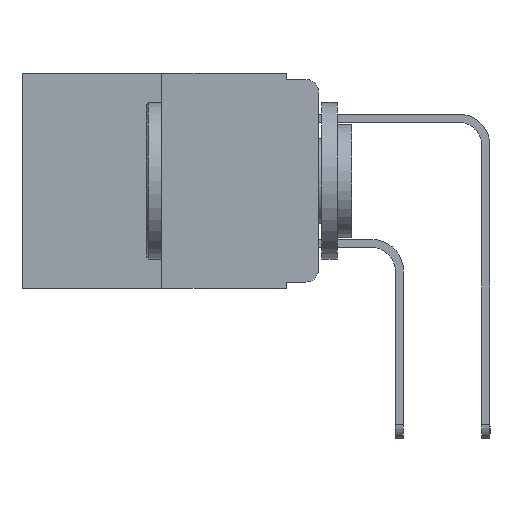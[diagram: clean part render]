
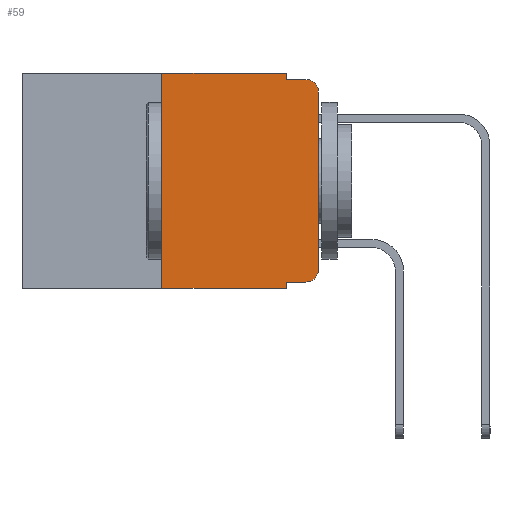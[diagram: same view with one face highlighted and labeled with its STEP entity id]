
A CAD part, left-side view. The second image highlights one B-rep face of the part: STEP entity #59.
In plain terms, the highlighted planar face has unit normal (-1, 0, 0).
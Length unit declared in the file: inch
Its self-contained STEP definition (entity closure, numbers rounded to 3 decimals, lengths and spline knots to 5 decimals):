
#59 = ADVANCED_FACE ( 'NONE', ( #5841 ), #3660, .F. ) ;
#407 = AXIS2_PLACEMENT_3D ( 'NONE', #15184, #13256, #22876 ) ;
#498 = CARTESIAN_POINT ( 'NONE',  ( 0., 0., -0.03 ) ) ;
#936 = CARTESIAN_POINT ( 'NONE',  ( 0., 0.02, -0.333 ) ) ;
#998 = DIRECTION ( 'NONE',  ( 0., 0., -1. ) ) ;
#1811 = EDGE_CURVE ( 'NONE', #6696, #3838, #9662, .T. ) ;
#2507 = CIRCLE ( 'NONE', #14789, 0.02 ) ;
#2534 = VERTEX_POINT ( 'NONE', #14826 ) ;
#2669 = CARTESIAN_POINT ( 'NONE',  ( 0., 0.051, 0. ) ) ;
#2766 = VERTEX_POINT ( 'NONE', #12106 ) ;
#3660 = PLANE ( 'NONE',  #18460 ) ;
#3807 = CARTESIAN_POINT ( 'NONE',  ( 0., 0.02, -0.313 ) ) ;
#3838 = VERTEX_POINT ( 'NONE', #12809 ) ;
#4015 = VECTOR ( 'NONE', #14456, 39.37008 ) ;
#4100 = ORIENTED_EDGE ( 'NONE', *, *, #6868, .T. ) ;
#4613 = VERTEX_POINT ( 'NONE', #936 ) ;
#4682 = CARTESIAN_POINT ( 'NONE',  ( 0., 0., -0.313 ) ) ;
#5069 = LINE ( 'NONE', #18771, #22053 ) ;
#5099 = EDGE_CURVE ( 'NONE', #6022, #4613, #18211, .T. ) ;
#5583 = EDGE_CURVE ( 'NONE', #6022, #3838, #8552, .T. ) ;
#5776 = VERTEX_POINT ( 'NONE', #4682 ) ;
#5841 = FACE_OUTER_BOUND ( 'NONE', #8766, .T. ) ;
#6022 = VERTEX_POINT ( 'NONE', #17378 ) ;
#6070 = LINE ( 'NONE', #13870, #11898 ) ;
#6507 = CARTESIAN_POINT ( 'NONE',  ( 0., 0.051, -0.01 ) ) ;
#6696 = VERTEX_POINT ( 'NONE', #12805 ) ;
#6868 = EDGE_CURVE ( 'NONE', #5776, #18580, #9602, .T. ) ;
#7466 = DIRECTION ( 'NONE',  ( 0., -1., 0. ) ) ;
#7610 = EDGE_CURVE ( 'NONE', #14787, #20910, #5069, .T. ) ;
#7739 = ORIENTED_EDGE ( 'NONE', *, *, #12053, .T. ) ;
#7995 = CARTESIAN_POINT ( 'NONE',  ( 0., 0.473, 0. ) ) ;
#8552 = LINE ( 'NONE', #2669, #16216 ) ;
#8599 = ORIENTED_EDGE ( 'NONE', *, *, #16244, .F. ) ;
#8720 = CARTESIAN_POINT ( 'NONE',  ( 0., 0.051, -0.333 ) ) ;
#8761 = CARTESIAN_POINT ( 'NONE',  ( 0., 0.051, 0. ) ) ;
#8766 = EDGE_LOOP ( 'NONE', ( #4100, #14458, #16681, #8599, #20989, #21946, #22911, #22703, #16181, #7739 ) ) ;
#9048 = CARTESIAN_POINT ( 'NONE',  ( 0., 0.051, 0. ) ) ;
#9602 = LINE ( 'NONE', #21250, #19546 ) ;
#9662 = LINE ( 'NONE', #23233, #20066 ) ;
#11454 = DIRECTION ( 'NONE',  ( 0., 0., -1. ) ) ;
#11843 = CIRCLE ( 'NONE', #407, 0.02 ) ;
#11898 = VECTOR ( 'NONE', #21705, 39.37008 ) ;
#12053 = EDGE_CURVE ( 'NONE', #4613, #5776, #2507, .T. ) ;
#12106 = CARTESIAN_POINT ( 'NONE',  ( 0., 0.051, -0.01 ) ) ;
#12388 = VECTOR ( 'NONE', #22313, 39.37008 ) ;
#12805 = CARTESIAN_POINT ( 'NONE',  ( 0., 0.25, -0.343 ) ) ;
#12809 = CARTESIAN_POINT ( 'NONE',  ( 0., 0.051, -0.343 ) ) ;
#13256 = DIRECTION ( 'NONE',  ( -1., 0., 0. ) ) ;
#13870 = CARTESIAN_POINT ( 'NONE',  ( 0., 0.25, 0. ) ) ;
#14456 = DIRECTION ( 'NONE',  ( 0., -1., 0. ) ) ;
#14458 = ORIENTED_EDGE ( 'NONE', *, *, #20421, .T. ) ;
#14543 = DIRECTION ( 'NONE',  ( 0., -1., 0. ) ) ;
#14787 = VERTEX_POINT ( 'NONE', #20457 ) ;
#14789 = AXIS2_PLACEMENT_3D ( 'NONE', #3807, #17881, #23779 ) ;
#14815 = LINE ( 'NONE', #9048, #19059 ) ;
#14826 = CARTESIAN_POINT ( 'NONE',  ( 0., 0.02, -0.01 ) ) ;
#15184 = CARTESIAN_POINT ( 'NONE',  ( 0., 0.02, -0.03 ) ) ;
#16181 = ORIENTED_EDGE ( 'NONE', *, *, #5099, .T. ) ;
#16216 = VECTOR ( 'NONE', #998, 39.37008 ) ;
#16244 = EDGE_CURVE ( 'NONE', #20910, #2766, #14815, .T. ) ;
#16505 = LINE ( 'NONE', #6507, #4015 ) ;
#16681 = ORIENTED_EDGE ( 'NONE', *, *, #18565, .F. ) ;
#17378 = CARTESIAN_POINT ( 'NONE',  ( 0., 0.051, -0.333 ) ) ;
#17881 = DIRECTION ( 'NONE',  ( -1., 0., 0. ) ) ;
#18211 = LINE ( 'NONE', #8720, #12388 ) ;
#18460 = AXIS2_PLACEMENT_3D ( 'NONE', #7995, #25323, #11454 ) ;
#18565 = EDGE_CURVE ( 'NONE', #2766, #2534, #16505, .T. ) ;
#18580 = VERTEX_POINT ( 'NONE', #498 ) ;
#18771 = CARTESIAN_POINT ( 'NONE',  ( 0., 0.473, 0. ) ) ;
#18962 = DIRECTION ( 'NONE',  ( 0., 0., 1. ) ) ;
#19059 = VECTOR ( 'NONE', #22638, 39.37008 ) ;
#19546 = VECTOR ( 'NONE', #18962, 39.37008 ) ;
#20066 = VECTOR ( 'NONE', #7466, 39.37008 ) ;
#20421 = EDGE_CURVE ( 'NONE', #18580, #2534, #11843, .T. ) ;
#20457 = CARTESIAN_POINT ( 'NONE',  ( 0., 0.25, 0. ) ) ;
#20910 = VERTEX_POINT ( 'NONE', #8761 ) ;
#20989 = ORIENTED_EDGE ( 'NONE', *, *, #7610, .F. ) ;
#21250 = CARTESIAN_POINT ( 'NONE',  ( 0., 0., 0. ) ) ;
#21705 = DIRECTION ( 'NONE',  ( 0., 0., 1. ) ) ;
#21946 = ORIENTED_EDGE ( 'NONE', *, *, #23307, .F. ) ;
#22053 = VECTOR ( 'NONE', #14543, 39.37008 ) ;
#22313 = DIRECTION ( 'NONE',  ( 0., -1., 0. ) ) ;
#22638 = DIRECTION ( 'NONE',  ( 0., 0., -1. ) ) ;
#22703 = ORIENTED_EDGE ( 'NONE', *, *, #5583, .F. ) ;
#22876 = DIRECTION ( 'NONE',  ( 0., 0., -1. ) ) ;
#22911 = ORIENTED_EDGE ( 'NONE', *, *, #1811, .T. ) ;
#23233 = CARTESIAN_POINT ( 'NONE',  ( 0., 0.473, -0.343 ) ) ;
#23307 = EDGE_CURVE ( 'NONE', #6696, #14787, #6070, .T. ) ;
#23779 = DIRECTION ( 'NONE',  ( 0., 0., -1. ) ) ;
#25323 = DIRECTION ( 'NONE',  ( 1., 0., 0. ) ) ;
